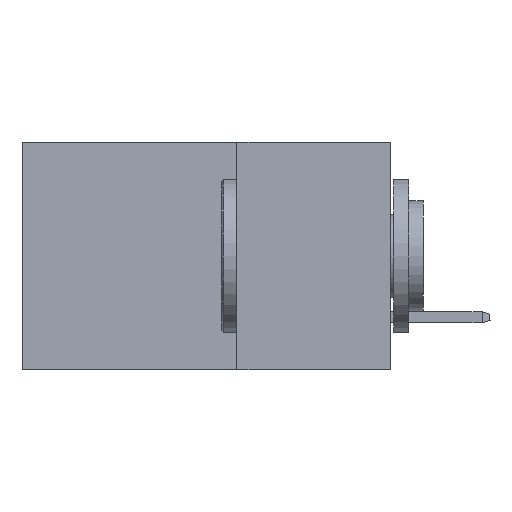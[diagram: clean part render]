
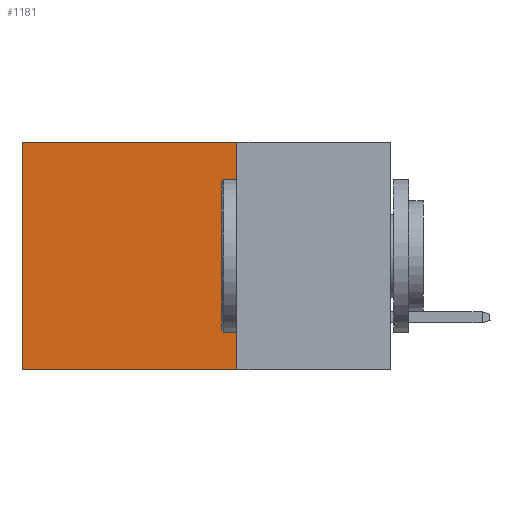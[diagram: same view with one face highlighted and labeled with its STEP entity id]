
A CAD part, left-side view. The second image highlights one B-rep face of the part: STEP entity #1181.
In plain terms, the highlighted planar face has unit normal (-1, 0, 0).
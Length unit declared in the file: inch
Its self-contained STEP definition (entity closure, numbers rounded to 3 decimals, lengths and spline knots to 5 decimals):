
#1181 = ADVANCED_FACE ( 'NONE', ( #15005 ), #3986, .F. ) ;
#1190 = DIRECTION ( 'NONE',  ( 0., 0., -1. ) ) ;
#1807 = LINE ( 'NONE', #33900, #10408 ) ;
#3986 = PLANE ( 'NONE',  #9851 ) ;
#4409 = VERTEX_POINT ( 'NONE', #33382 ) ;
#5293 = DIRECTION ( 'NONE',  ( 0., 1., 0. ) ) ;
#8298 = EDGE_LOOP ( 'NONE', ( #12981, #21045, #26160, #19816 ) ) ;
#9273 = CARTESIAN_POINT ( 'NONE',  ( 0.2875, 0.6, 0. ) ) ;
#9851 = AXIS2_PLACEMENT_3D ( 'NONE', #35640, #18312, #1190 ) ;
#10204 = VECTOR ( 'NONE', #10227, 39.37008 ) ;
#10227 = DIRECTION ( 'NONE',  ( 0., 1., 0. ) ) ;
#10408 = VECTOR ( 'NONE', #5293, 39.37008 ) ;
#12556 = EDGE_CURVE ( 'NONE', #21788, #21661, #1807, .T. ) ;
#12981 = ORIENTED_EDGE ( 'NONE', *, *, #30187, .T. ) ;
#15005 = FACE_OUTER_BOUND ( 'NONE', #8298, .T. ) ;
#15951 = CARTESIAN_POINT ( 'NONE',  ( 0.2875, 0.25, 0. ) ) ;
#16087 = LINE ( 'NONE', #9273, #24641 ) ;
#16856 = CARTESIAN_POINT ( 'NONE',  ( 0.2875, 0.25, 0. ) ) ;
#18312 = DIRECTION ( 'NONE',  ( 1., 0., 0. ) ) ;
#18398 = EDGE_CURVE ( 'NONE', #21788, #23524, #25616, .T. ) ;
#19816 = ORIENTED_EDGE ( 'NONE', *, *, #12556, .T. ) ;
#21045 = ORIENTED_EDGE ( 'NONE', *, *, #32956, .F. ) ;
#21661 = VERTEX_POINT ( 'NONE', #27180 ) ;
#21788 = VERTEX_POINT ( 'NONE', #16856 ) ;
#23524 = VERTEX_POINT ( 'NONE', #24531 ) ;
#24531 = CARTESIAN_POINT ( 'NONE',  ( 0.2875, 0.25, -0.37 ) ) ;
#24641 = VECTOR ( 'NONE', #32169, 39.37008 ) ;
#25616 = LINE ( 'NONE', #15951, #33306 ) ;
#26160 = ORIENTED_EDGE ( 'NONE', *, *, #18398, .F. ) ;
#27180 = CARTESIAN_POINT ( 'NONE',  ( 0.2875, 0.6, 0. ) ) ;
#30187 = EDGE_CURVE ( 'NONE', #21661, #4409, #16087, .T. ) ;
#32169 = DIRECTION ( 'NONE',  ( 0., 0., -1. ) ) ;
#32956 = EDGE_CURVE ( 'NONE', #23524, #4409, #33054, .T. ) ;
#33054 = LINE ( 'NONE', #35935, #10204 ) ;
#33306 = VECTOR ( 'NONE', #36132, 39.37008 ) ;
#33382 = CARTESIAN_POINT ( 'NONE',  ( 0.2875, 0.6, -0.37 ) ) ;
#33900 = CARTESIAN_POINT ( 'NONE',  ( 0.2875, 0.25, 0. ) ) ;
#35640 = CARTESIAN_POINT ( 'NONE',  ( 0.2875, 0.25, 0. ) ) ;
#35935 = CARTESIAN_POINT ( 'NONE',  ( 0.2875, 0.25, -0.37 ) ) ;
#36132 = DIRECTION ( 'NONE',  ( 0., 0., -1. ) ) ;
